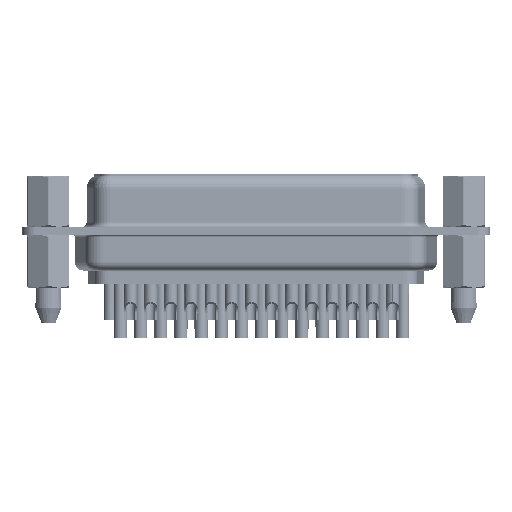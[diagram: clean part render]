
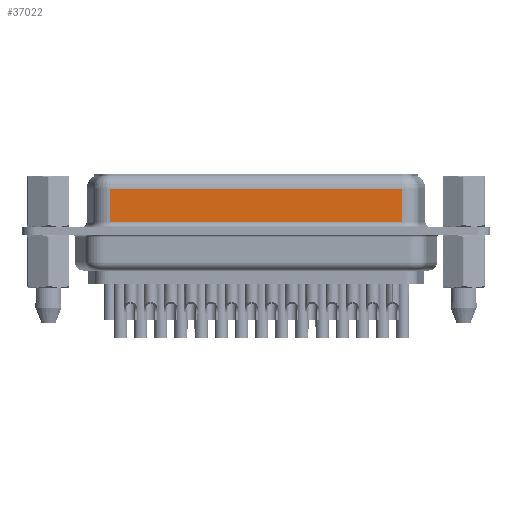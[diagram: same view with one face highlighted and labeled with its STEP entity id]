
A CAD part, front view. The second image highlights one B-rep face of the part: STEP entity #37022.
In plain terms, the highlighted planar face has unit normal (0, -1, 0).
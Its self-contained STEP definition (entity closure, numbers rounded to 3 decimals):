
#125 = VECTOR ( 'NONE', #28928, 1000. ) ;
#1525 = LINE ( 'NONE', #2137, #5840 ) ;
#2060 = CARTESIAN_POINT ( 'NONE',  ( 7.008, -3.95, 6.45 ) ) ;
#2119 = ORIENTED_EDGE ( 'NONE', *, *, #38897, .T. ) ;
#2137 = CARTESIAN_POINT ( 'NONE',  ( 40.032, -3.95, 0.95 ) ) ;
#3652 = ORIENTED_EDGE ( 'NONE', *, *, #36328, .T. ) ;
#3819 = ORIENTED_EDGE ( 'NONE', *, *, #32568, .T. ) ;
#5078 = DIRECTION ( 'NONE',  ( 0., 0., -1. ) ) ;
#5470 = LINE ( 'NONE', #2060, #8822 ) ;
#5840 = VECTOR ( 'NONE', #27885, 1000. ) ;
#5842 = CARTESIAN_POINT ( 'NONE',  ( 7.008, -3.95, 0.95 ) ) ;
#7636 = CARTESIAN_POINT ( 'NONE',  ( 7.008, -3.95, 4.7 ) ) ;
#7914 = VERTEX_POINT ( 'NONE', #5842 ) ;
#8822 = VECTOR ( 'NONE', #38013, 1000. ) ;
#11157 = PLANE ( 'NONE',  #25161 ) ;
#11623 = CARTESIAN_POINT ( 'NONE',  ( 40.032, -3.95, 4.7 ) ) ;
#11944 = CARTESIAN_POINT ( 'NONE',  ( 40.032, -3.95, 4.7 ) ) ;
#14852 = VECTOR ( 'NONE', #5078, 1000. ) ;
#15142 = LINE ( 'NONE', #11944, #125 ) ;
#17556 = FACE_OUTER_BOUND ( 'NONE', #28828, .T. ) ;
#23922 = CARTESIAN_POINT ( 'NONE',  ( 40.032, -3.95, 6.45 ) ) ;
#24121 = DIRECTION ( 'NONE',  ( 0., 1., 0. ) ) ;
#24318 = DIRECTION ( 'NONE',  ( 0., 0., 1. ) ) ;
#25161 = AXIS2_PLACEMENT_3D ( 'NONE', #23922, #24121, #24318 ) ;
#27215 = CARTESIAN_POINT ( 'NONE',  ( 40.032, -3.95, 6.45 ) ) ;
#27885 = DIRECTION ( 'NONE',  ( 1., 0., 0. ) ) ;
#28828 = EDGE_LOOP ( 'NONE', ( #36733, #2119, #3652, #3819 ) ) ;
#28928 = DIRECTION ( 'NONE',  ( -1., 0., 0. ) ) ;
#29956 = VERTEX_POINT ( 'NONE', #40927 ) ;
#32568 = EDGE_CURVE ( 'NONE', #7914, #29956, #1525, .T. ) ;
#33104 = EDGE_CURVE ( 'NONE', #36679, #29956, #34221, .T. ) ;
#34221 = LINE ( 'NONE', #27215, #14852 ) ;
#36328 = EDGE_CURVE ( 'NONE', #40226, #7914, #5470, .T. ) ;
#36679 = VERTEX_POINT ( 'NONE', #11623 ) ;
#36733 = ORIENTED_EDGE ( 'NONE', *, *, #33104, .F. ) ;
#37022 = ADVANCED_FACE ( 'NONE', ( #17556 ), #11157, .F. ) ;
#38013 = DIRECTION ( 'NONE',  ( 0., 0., -1. ) ) ;
#38897 = EDGE_CURVE ( 'NONE', #36679, #40226, #15142, .T. ) ;
#40226 = VERTEX_POINT ( 'NONE', #7636 ) ;
#40927 = CARTESIAN_POINT ( 'NONE',  ( 40.032, -3.95, 0.95 ) ) ;
